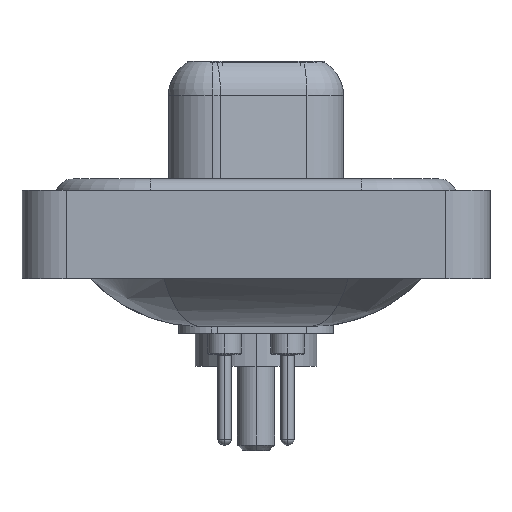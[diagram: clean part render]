
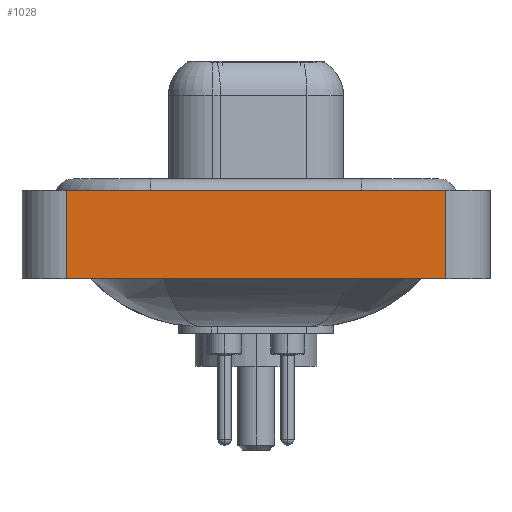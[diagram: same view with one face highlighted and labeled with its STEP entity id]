
A CAD part, left-side view. The second image highlights one B-rep face of the part: STEP entity #1028.
In plain terms, the highlighted planar face has unit normal (-1, 0, 0).
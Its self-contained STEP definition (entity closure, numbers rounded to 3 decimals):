
#602 = ORIENTED_EDGE ( 'NONE', *, *, #8284, .F. ) ;
#1028 = ADVANCED_FACE ( 'NONE', ( #19040 ), #7332, .T. ) ;
#1063 = VERTEX_POINT ( 'NONE', #10588 ) ;
#2523 = DIRECTION ( 'NONE',  ( 0., 0., 1. ) ) ;
#3759 = DIRECTION ( 'NONE',  ( 0., 0., 1. ) ) ;
#3946 = DIRECTION ( 'NONE',  ( 0., -1., 0. ) ) ;
#4585 = DIRECTION ( 'NONE',  ( 0., 0., 1. ) ) ;
#5592 = EDGE_CURVE ( 'NONE', #1063, #19518, #11883, .T. ) ;
#5837 = EDGE_CURVE ( 'NONE', #7791, #19518, #7958, .T. ) ;
#7332 = PLANE ( 'NONE',  #7401 ) ;
#7401 = AXIS2_PLACEMENT_3D ( 'NONE', #12261, #18710, #3759 ) ;
#7440 = CARTESIAN_POINT ( 'NONE',  ( -7.3, 8.55, -3.6 ) ) ;
#7791 = VERTEX_POINT ( 'NONE', #21040 ) ;
#7876 = LINE ( 'NONE', #21439, #19657 ) ;
#7958 = LINE ( 'NONE', #14534, #21758 ) ;
#8284 = EDGE_CURVE ( 'NONE', #14942, #1063, #21466, .T. ) ;
#9149 = VECTOR ( 'NONE', #20542, 1000. ) ;
#10219 = EDGE_CURVE ( 'NONE', #14942, #7791, #7876, .T. ) ;
#10351 = EDGE_LOOP ( 'NONE', ( #14208, #21517, #602, #18047 ) ) ;
#10588 = CARTESIAN_POINT ( 'NONE',  ( -7.3, 8.55, 0.4 ) ) ;
#11883 = LINE ( 'NONE', #17100, #9149 ) ;
#12261 = CARTESIAN_POINT ( 'NONE',  ( -7.3, -8.55, -3.6 ) ) ;
#13376 = CARTESIAN_POINT ( 'NONE',  ( -7.3, -8.55, 0.4 ) ) ;
#14208 = ORIENTED_EDGE ( 'NONE', *, *, #5837, .T. ) ;
#14534 = CARTESIAN_POINT ( 'NONE',  ( -7.3, -8.55, -3.6 ) ) ;
#14942 = VERTEX_POINT ( 'NONE', #7440 ) ;
#16136 = CARTESIAN_POINT ( 'NONE',  ( -7.3, 8.55, -3.6 ) ) ;
#16900 = VECTOR ( 'NONE', #2523, 1000. ) ;
#17100 = CARTESIAN_POINT ( 'NONE',  ( -7.3, -8.55, 0.4 ) ) ;
#18047 = ORIENTED_EDGE ( 'NONE', *, *, #10219, .T. ) ;
#18710 = DIRECTION ( 'NONE',  ( -1., 0., 0. ) ) ;
#19040 = FACE_OUTER_BOUND ( 'NONE', #10351, .T. ) ;
#19518 = VERTEX_POINT ( 'NONE', #13376 ) ;
#19657 = VECTOR ( 'NONE', #3946, 1000. ) ;
#20542 = DIRECTION ( 'NONE',  ( 0., -1., 0. ) ) ;
#21040 = CARTESIAN_POINT ( 'NONE',  ( -7.3, -8.55, -3.6 ) ) ;
#21439 = CARTESIAN_POINT ( 'NONE',  ( -7.3, -8.55, -3.6 ) ) ;
#21466 = LINE ( 'NONE', #16136, #16900 ) ;
#21517 = ORIENTED_EDGE ( 'NONE', *, *, #5592, .F. ) ;
#21758 = VECTOR ( 'NONE', #4585, 1000. ) ;
